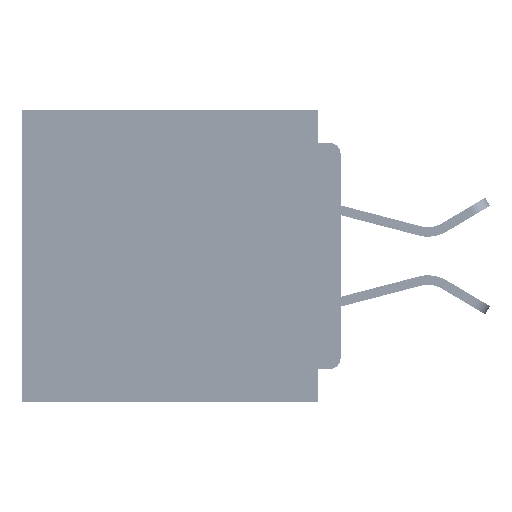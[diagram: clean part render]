
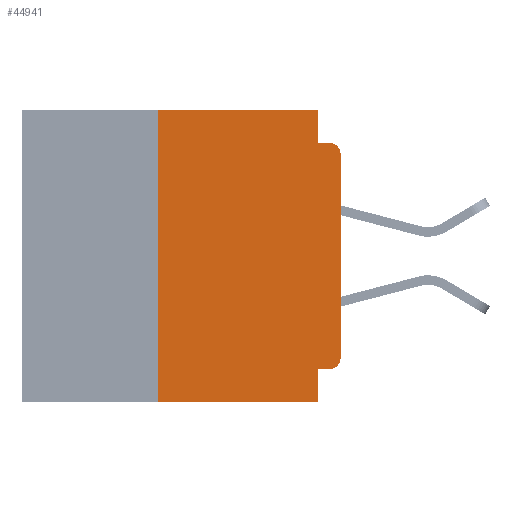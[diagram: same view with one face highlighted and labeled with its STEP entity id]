
A CAD part, left-side view. The second image highlights one B-rep face of the part: STEP entity #44941.
In plain terms, the highlighted planar face has unit normal (-1, 0, 0).
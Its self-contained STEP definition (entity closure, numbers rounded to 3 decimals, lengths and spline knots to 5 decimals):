
#2 = CARTESIAN_POINT ( 'NONE',  ( 0., 0.015, -0.34 ) ) ;
#19 = CIRCLE ( 'NONE', #49769, 0.015 ) ;
#145 = AXIS2_PLACEMENT_3D ( 'NONE', #5230, #47056, #19229 ) ;
#305 = DIRECTION ( 'NONE',  ( 0., -1., 0. ) ) ;
#377 = VERTEX_POINT ( 'NONE', #38074 ) ;
#391 = ORIENTED_EDGE ( 'NONE', *, *, #43910, .F. ) ;
#511 = CARTESIAN_POINT ( 'NONE',  ( 0., 0.437, -0.4 ) ) ;
#1112 = ORIENTED_EDGE ( 'NONE', *, *, #12870, .F. ) ;
#2055 = DIRECTION ( 'NONE',  ( 0., 0., -1. ) ) ;
#3380 = CARTESIAN_POINT ( 'NONE',  ( 0., 0.25, 0. ) ) ;
#4744 = DIRECTION ( 'NONE',  ( 0., 0., -1. ) ) ;
#5230 = CARTESIAN_POINT ( 'NONE',  ( 0., 0.437, 0. ) ) ;
#5737 = CARTESIAN_POINT ( 'NONE',  ( 0., 0.437, 0. ) ) ;
#5795 = ORIENTED_EDGE ( 'NONE', *, *, #43651, .T. ) ;
#6011 = CARTESIAN_POINT ( 'NONE',  ( 0., 0.25, -0.4 ) ) ;
#6295 = CARTESIAN_POINT ( 'NONE',  ( 0., 0.031, -0.045 ) ) ;
#6465 = ORIENTED_EDGE ( 'NONE', *, *, #9994, .T. ) ;
#7160 = EDGE_CURVE ( 'NONE', #36292, #53022, #57822, .T. ) ;
#7294 = VECTOR ( 'NONE', #26700, 39.37008 ) ;
#7407 = VERTEX_POINT ( 'NONE', #15631 ) ;
#7621 = CARTESIAN_POINT ( 'NONE',  ( 0., 0., -0.355 ) ) ;
#9008 = CARTESIAN_POINT ( 'NONE',  ( 0., 0., 0. ) ) ;
#9074 = CARTESIAN_POINT ( 'NONE',  ( 0., 0.031, -0.355 ) ) ;
#9994 = EDGE_CURVE ( 'NONE', #18583, #377, #25062, .T. ) ;
#10368 = EDGE_LOOP ( 'NONE', ( #21793, #52416, #15245, #391, #1112, #34111, #6465, #14214, #46572, #5795 ) ) ;
#10766 = EDGE_CURVE ( 'NONE', #17914, #34202, #15439, .T. ) ;
#11748 = EDGE_CURVE ( 'NONE', #53022, #34202, #19, .T. ) ;
#12870 = EDGE_CURVE ( 'NONE', #49975, #7407, #36322, .T. ) ;
#13432 = DIRECTION ( 'NONE',  ( 0., 0., 1. ) ) ;
#14214 = ORIENTED_EDGE ( 'NONE', *, *, #58986, .F. ) ;
#15245 = ORIENTED_EDGE ( 'NONE', *, *, #10766, .F. ) ;
#15439 = LINE ( 'NONE', #24674, #41693 ) ;
#15544 = CARTESIAN_POINT ( 'NONE',  ( 0., 0.015, -0.06 ) ) ;
#15631 = CARTESIAN_POINT ( 'NONE',  ( 0., 0.031, 0. ) ) ;
#15886 = VECTOR ( 'NONE', #48168, 39.37008 ) ;
#17914 = VERTEX_POINT ( 'NONE', #6295 ) ;
#18101 = CIRCLE ( 'NONE', #34089, 0.015 ) ;
#18494 = LINE ( 'NONE', #43980, #40373 ) ;
#18583 = VERTEX_POINT ( 'NONE', #6011 ) ;
#19229 = DIRECTION ( 'NONE',  ( 0., 0., -1. ) ) ;
#19636 = LINE ( 'NONE', #54346, #7294 ) ;
#20261 = DIRECTION ( 'NONE',  ( 0., 0., -1. ) ) ;
#21276 = FACE_OUTER_BOUND ( 'NONE', #10368, .T. ) ;
#21793 = ORIENTED_EDGE ( 'NONE', *, *, #7160, .T. ) ;
#24233 = DIRECTION ( 'NONE',  ( 0., -1., 0. ) ) ;
#24674 = CARTESIAN_POINT ( 'NONE',  ( 0., 0., -0.045 ) ) ;
#25044 = CARTESIAN_POINT ( 'NONE',  ( 0., 0.031, 0. ) ) ;
#25062 = LINE ( 'NONE', #511, #48285 ) ;
#26700 = DIRECTION ( 'NONE',  ( 0., 0., 1. ) ) ;
#26984 = CARTESIAN_POINT ( 'NONE',  ( 0., 0.015, -0.355 ) ) ;
#30479 = EDGE_CURVE ( 'NONE', #18583, #49975, #19636, .T. ) ;
#31229 = LINE ( 'NONE', #25044, #15886 ) ;
#32615 = DIRECTION ( 'NONE',  ( -1., 0., 0. ) ) ;
#32740 = CARTESIAN_POINT ( 'NONE',  ( 0., 0.015, -0.045 ) ) ;
#33247 = EDGE_CURVE ( 'NONE', #35506, #39221, #49173, .T. ) ;
#34089 = AXIS2_PLACEMENT_3D ( 'NONE', #2, #32615, #4744 ) ;
#34111 = ORIENTED_EDGE ( 'NONE', *, *, #30479, .F. ) ;
#34202 = VERTEX_POINT ( 'NONE', #32740 ) ;
#35469 = DIRECTION ( 'NONE',  ( 0., 1., 0. ) ) ;
#35506 = VERTEX_POINT ( 'NONE', #26984 ) ;
#36292 = VERTEX_POINT ( 'NONE', #42968 ) ;
#36322 = LINE ( 'NONE', #5737, #59342 ) ;
#36898 = VECTOR ( 'NONE', #35469, 39.37008 ) ;
#38074 = CARTESIAN_POINT ( 'NONE',  ( 0., 0.031, -0.4 ) ) ;
#39221 = VERTEX_POINT ( 'NONE', #9074 ) ;
#40373 = VECTOR ( 'NONE', #2055, 39.37008 ) ;
#41693 = VECTOR ( 'NONE', #52391, 39.37008 ) ;
#42445 = PLANE ( 'NONE',  #145 ) ;
#42968 = CARTESIAN_POINT ( 'NONE',  ( 0., 0., -0.34 ) ) ;
#43651 = EDGE_CURVE ( 'NONE', #35506, #36292, #18101, .T. ) ;
#43910 = EDGE_CURVE ( 'NONE', #7407, #17914, #31229, .T. ) ;
#43980 = CARTESIAN_POINT ( 'NONE',  ( 0., 0.031, -0.4 ) ) ;
#44941 = ADVANCED_FACE ( 'NONE', ( #21276 ), #42445, .F. ) ;
#46572 = ORIENTED_EDGE ( 'NONE', *, *, #33247, .F. ) ;
#47056 = DIRECTION ( 'NONE',  ( 1., 0., 0. ) ) ;
#47643 = CARTESIAN_POINT ( 'NONE',  ( 0., 0., -0.06 ) ) ;
#48062 = DIRECTION ( 'NONE',  ( -1., 0., 0. ) ) ;
#48168 = DIRECTION ( 'NONE',  ( 0., 0., -1. ) ) ;
#48285 = VECTOR ( 'NONE', #305, 39.37008 ) ;
#49173 = LINE ( 'NONE', #7621, #36898 ) ;
#49769 = AXIS2_PLACEMENT_3D ( 'NONE', #15544, #48062, #20261 ) ;
#49975 = VERTEX_POINT ( 'NONE', #3380 ) ;
#52391 = DIRECTION ( 'NONE',  ( 0., -1., 0. ) ) ;
#52416 = ORIENTED_EDGE ( 'NONE', *, *, #11748, .T. ) ;
#53022 = VERTEX_POINT ( 'NONE', #47643 ) ;
#54346 = CARTESIAN_POINT ( 'NONE',  ( 0., 0.25, -0.4 ) ) ;
#56404 = VECTOR ( 'NONE', #13432, 39.37008 ) ;
#57822 = LINE ( 'NONE', #9008, #56404 ) ;
#58986 = EDGE_CURVE ( 'NONE', #39221, #377, #18494, .T. ) ;
#59342 = VECTOR ( 'NONE', #24233, 39.37008 ) ;
